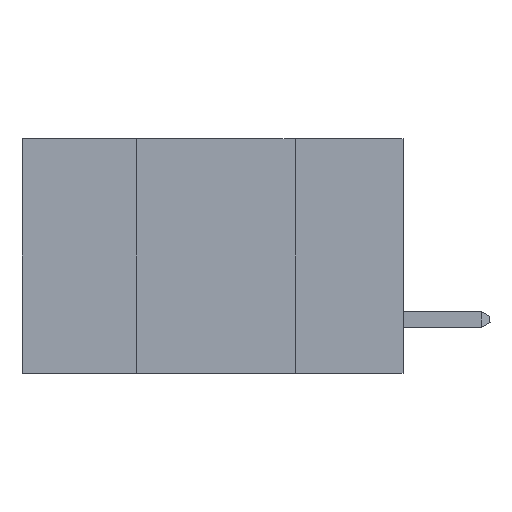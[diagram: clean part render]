
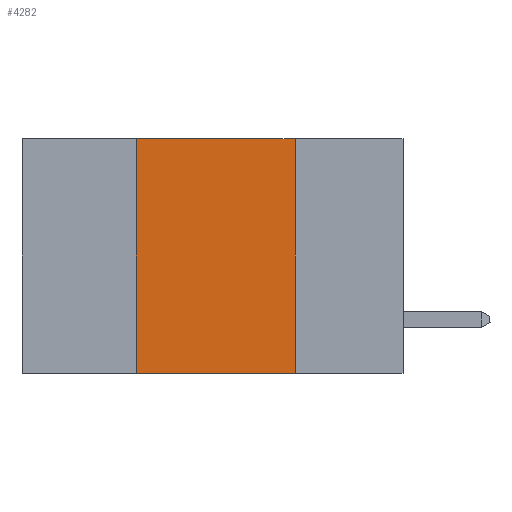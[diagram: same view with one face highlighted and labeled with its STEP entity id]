
A CAD part, left-side view. The second image highlights one B-rep face of the part: STEP entity #4282.
In plain terms, the highlighted planar face has unit normal (-1, 0, 0).
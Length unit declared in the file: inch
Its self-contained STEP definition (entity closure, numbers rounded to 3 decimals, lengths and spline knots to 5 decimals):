
#137 = VECTOR ( 'NONE', #12652, 39.37008 ) ;
#181 = VECTOR ( 'NONE', #23749, 39.37008 ) ;
#698 = ORIENTED_EDGE ( 'NONE', *, *, #12242, .T. ) ;
#864 = VERTEX_POINT ( 'NONE', #8518 ) ;
#2456 = LINE ( 'NONE', #22894, #137 ) ;
#3287 = AXIS2_PLACEMENT_3D ( 'NONE', #16652, #13215, #4905 ) ;
#3371 = ORIENTED_EDGE ( 'NONE', *, *, #7637, .F. ) ;
#4282 = ADVANCED_FACE ( 'NONE', ( #20951 ), #8163, .F. ) ;
#4905 = DIRECTION ( 'NONE',  ( 0., 0., -1. ) ) ;
#5648 = DIRECTION ( 'NONE',  ( 0., 0., -1. ) ) ;
#6315 = EDGE_CURVE ( 'NONE', #16299, #6385, #18658, .T. ) ;
#6385 = VERTEX_POINT ( 'NONE', #19625 ) ;
#7637 = EDGE_CURVE ( 'NONE', #864, #9364, #18586, .T. ) ;
#8163 = PLANE ( 'NONE',  #3287 ) ;
#8518 = CARTESIAN_POINT ( 'NONE',  ( 0., 0.17, 0. ) ) ;
#9364 = VERTEX_POINT ( 'NONE', #24938 ) ;
#10776 = ORIENTED_EDGE ( 'NONE', *, *, #26978, .F. ) ;
#12242 = EDGE_CURVE ( 'NONE', #16299, #9364, #2456, .T. ) ;
#12339 = VECTOR ( 'NONE', #5648, 39.37008 ) ;
#12652 = DIRECTION ( 'NONE',  ( 0., -1., 0. ) ) ;
#13215 = DIRECTION ( 'NONE',  ( 1., 0., 0. ) ) ;
#13414 = CARTESIAN_POINT ( 'NONE',  ( 0., 0.6, 0. ) ) ;
#14292 = VECTOR ( 'NONE', #25703, 39.37008 ) ;
#15289 = CARTESIAN_POINT ( 'NONE',  ( 0., 0.17, 0. ) ) ;
#16299 = VERTEX_POINT ( 'NONE', #21304 ) ;
#16652 = CARTESIAN_POINT ( 'NONE',  ( 0., 0.6, 0. ) ) ;
#17854 = LINE ( 'NONE', #13414, #14292 ) ;
#18586 = LINE ( 'NONE', #15289, #12339 ) ;
#18658 = LINE ( 'NONE', #25690, #181 ) ;
#19625 = CARTESIAN_POINT ( 'NONE',  ( 0., 0.42, 0. ) ) ;
#20951 = FACE_OUTER_BOUND ( 'NONE', #24821, .T. ) ;
#21304 = CARTESIAN_POINT ( 'NONE',  ( 0., 0.42, -0.37 ) ) ;
#22894 = CARTESIAN_POINT ( 'NONE',  ( 0., 0.6, -0.37 ) ) ;
#23749 = DIRECTION ( 'NONE',  ( 0., 0., 1. ) ) ;
#24821 = EDGE_LOOP ( 'NONE', ( #3371, #10776, #25607, #698 ) ) ;
#24938 = CARTESIAN_POINT ( 'NONE',  ( 0., 0.17, -0.37 ) ) ;
#25607 = ORIENTED_EDGE ( 'NONE', *, *, #6315, .F. ) ;
#25690 = CARTESIAN_POINT ( 'NONE',  ( 0., 0.42, 0. ) ) ;
#25703 = DIRECTION ( 'NONE',  ( 0., -1., 0. ) ) ;
#26978 = EDGE_CURVE ( 'NONE', #6385, #864, #17854, .T. ) ;
